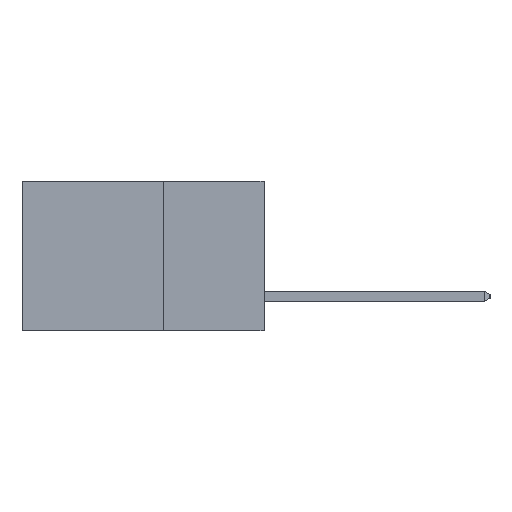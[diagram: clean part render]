
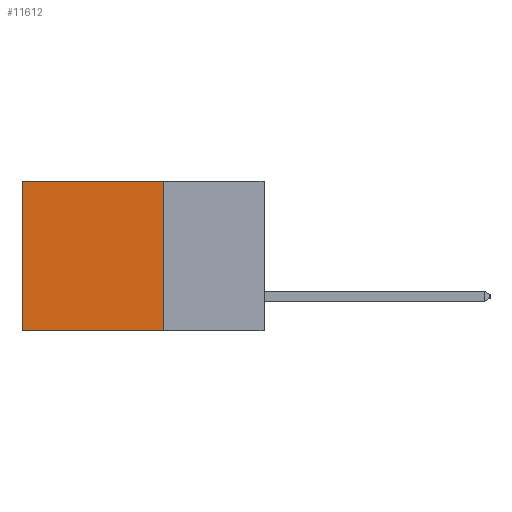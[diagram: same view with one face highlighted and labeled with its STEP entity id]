
A CAD part, left-side view. The second image highlights one B-rep face of the part: STEP entity #11612.
In plain terms, the highlighted planar face has unit normal (-1, 0, 0).
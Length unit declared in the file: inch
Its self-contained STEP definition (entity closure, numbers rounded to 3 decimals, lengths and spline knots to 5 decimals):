
#241 = VECTOR ( 'NONE', #8429, 39.37008 ) ;
#272 = LINE ( 'NONE', #3125, #5511 ) ;
#597 = CARTESIAN_POINT ( 'NONE',  ( 0.2615, 0.25, -0.37 ) ) ;
#1221 = VERTEX_POINT ( 'NONE', #11959 ) ;
#1485 = EDGE_LOOP ( 'NONE', ( #11401, #10864, #9306, #10344 ) ) ;
#1674 = DIRECTION ( 'NONE',  ( 0., 0., -1. ) ) ;
#1814 = CARTESIAN_POINT ( 'NONE',  ( 0.2615, 0.25, -0.37 ) ) ;
#2853 = VERTEX_POINT ( 'NONE', #1814 ) ;
#3125 = CARTESIAN_POINT ( 'NONE',  ( 0.2615, 0.6, -0.37 ) ) ;
#3482 = CARTESIAN_POINT ( 'NONE',  ( 0.2615, 0.25, -0.37 ) ) ;
#3526 = PLANE ( 'NONE',  #4903 ) ;
#3948 = EDGE_CURVE ( 'NONE', #7447, #1221, #272, .T. ) ;
#4301 = CARTESIAN_POINT ( 'NONE',  ( 0.2615, 0.6, 0. ) ) ;
#4564 = DIRECTION ( 'NONE',  ( 0., 0., -1. ) ) ;
#4903 = AXIS2_PLACEMENT_3D ( 'NONE', #3482, #10662, #4564 ) ;
#5136 = VERTEX_POINT ( 'NONE', #10852 ) ;
#5324 = EDGE_CURVE ( 'NONE', #5136, #7447, #8233, .T. ) ;
#5511 = VECTOR ( 'NONE', #10501, 39.37008 ) ;
#5835 = VECTOR ( 'NONE', #6868, 39.37008 ) ;
#6868 = DIRECTION ( 'NONE',  ( 0., 1., 0. ) ) ;
#7447 = VERTEX_POINT ( 'NONE', #4301 ) ;
#8016 = FACE_OUTER_BOUND ( 'NONE', #1485, .T. ) ;
#8233 = LINE ( 'NONE', #11671, #241 ) ;
#8314 = EDGE_CURVE ( 'NONE', #2853, #1221, #8579, .T. ) ;
#8429 = DIRECTION ( 'NONE',  ( 0., 1., 0. ) ) ;
#8506 = VECTOR ( 'NONE', #1674, 39.37008 ) ;
#8579 = LINE ( 'NONE', #10900, #5835 ) ;
#8832 = LINE ( 'NONE', #597, #8506 ) ;
#9306 = ORIENTED_EDGE ( 'NONE', *, *, #11782, .F. ) ;
#10344 = ORIENTED_EDGE ( 'NONE', *, *, #5324, .T. ) ;
#10501 = DIRECTION ( 'NONE',  ( 0., 0., -1. ) ) ;
#10662 = DIRECTION ( 'NONE',  ( 1., 0., 0. ) ) ;
#10852 = CARTESIAN_POINT ( 'NONE',  ( 0.2615, 0.25, 0. ) ) ;
#10864 = ORIENTED_EDGE ( 'NONE', *, *, #8314, .F. ) ;
#10900 = CARTESIAN_POINT ( 'NONE',  ( 0.2615, 0.25, -0.37 ) ) ;
#11401 = ORIENTED_EDGE ( 'NONE', *, *, #3948, .T. ) ;
#11612 = ADVANCED_FACE ( 'NONE', ( #8016 ), #3526, .F. ) ;
#11671 = CARTESIAN_POINT ( 'NONE',  ( 0.2615, 0.25, 0. ) ) ;
#11782 = EDGE_CURVE ( 'NONE', #5136, #2853, #8832, .T. ) ;
#11959 = CARTESIAN_POINT ( 'NONE',  ( 0.2615, 0.6, -0.37 ) ) ;
